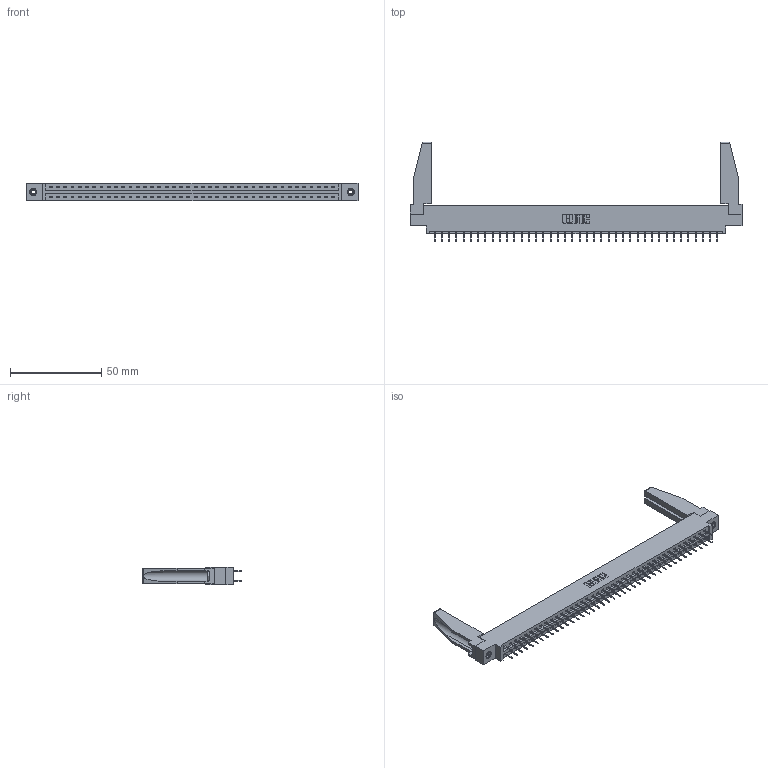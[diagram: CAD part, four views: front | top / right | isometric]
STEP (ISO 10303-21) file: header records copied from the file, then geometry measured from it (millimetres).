
FILE_DESCRIPTION (( 'STEP AP203' ), '1' );
FILE_NAME ('387-080-524-878.STEP', '2019-10-22T08:19:18', ( '' ), ( '' ), 'SwSTEP 2.0', 'SolidWorks 2016', '' );
FILE_SCHEMA (( 'CONFIG_CONTROL_DESIGN' ));
Length unit declared in the file: inch
Products named in the file (5): 345-250-001_345-250-001-102; 345-292-001_345-293-124; 337 Part_0.170 Offset - 0.156 Dia-TI; 307-220-078; 387-080-524-878
Assembly tree (85 placements, depth 2):
  387-080-524-878
    337 Part_0.170 Offset - 0.156 Dia-TI
    345-292-001_345-293-124  x80
    345-250-001_345-250-001-102  x2
    307-220-078  x2
Bounding box: 181.51 x 54.49 x 9.4 mm (x, y, z)
Volume: 22856.9 mm3; surface area: 24869.2 mm2
Topology: 85 solids, 85 shells, 4888 faces, 13853 edges, 8906 vertices
Faces by surface type: plane 3678, cylinder 1194, cone 12, torus 4
Entity records: 33918 total; most frequent: CARTESIAN_POINT 5716, ORIENTED_EDGE 5608, DIRECTION 4872, EDGE_CURVE 2804, VECTOR 2642, LINE 2642, VERTEX_POINT 1860, AXIS2_PLACEMENT_3D 1115
